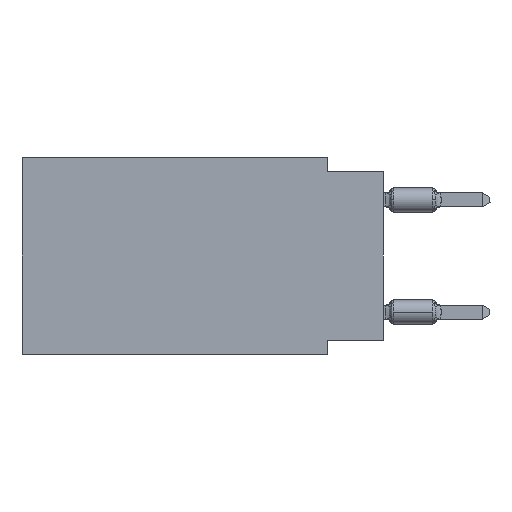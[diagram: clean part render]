
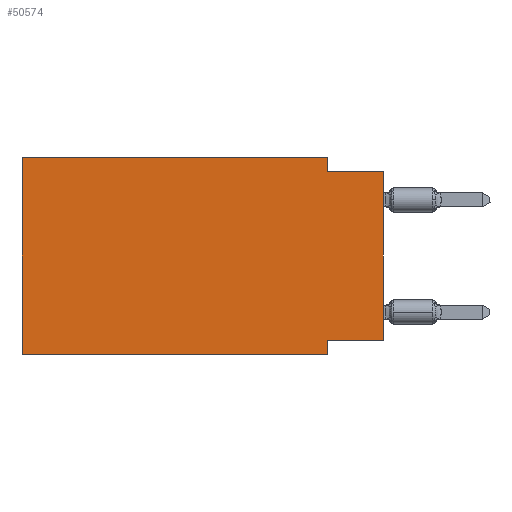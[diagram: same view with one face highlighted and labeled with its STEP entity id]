
A CAD part, left-side view. The second image highlights one B-rep face of the part: STEP entity #50574.
In plain terms, the highlighted planar face has unit normal (-1, 0, 0).
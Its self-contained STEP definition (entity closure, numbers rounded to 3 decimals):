
#2244 = VECTOR ( 'NONE', #19840, 1000. ) ;
#3026 = AXIS2_PLACEMENT_3D ( 'NONE', #25866, #55266, #50048 ) ;
#5818 = VERTEX_POINT ( 'NONE', #38947 ) ;
#6090 = DIRECTION ( 'NONE',  ( 0., 0., -1. ) ) ;
#6147 = ORIENTED_EDGE ( 'NONE', *, *, #39182, .F. ) ;
#7715 = EDGE_CURVE ( 'NONE', #68436, #34919, #61550, .T. ) ;
#7778 = VERTEX_POINT ( 'NONE', #38865 ) ;
#8231 = EDGE_CURVE ( 'NONE', #7778, #45000, #68686, .T. ) ;
#8926 = LINE ( 'NONE', #21599, #73499 ) ;
#9956 = CARTESIAN_POINT ( 'NONE',  ( 0., 0., -8.255 ) ) ;
#10507 = DIRECTION ( 'NONE',  ( 0., 1., 0. ) ) ;
#10569 = LINE ( 'NONE', #57133, #27972 ) ;
#10819 = LINE ( 'NONE', #20940, #14606 ) ;
#11310 = EDGE_CURVE ( 'NONE', #34919, #45000, #65997, .T. ) ;
#12389 = CARTESIAN_POINT ( 'NONE',  ( 0., 0., -0.635 ) ) ;
#12663 = VECTOR ( 'NONE', #46762, 1000. ) ;
#14606 = VECTOR ( 'NONE', #15705, 1000. ) ;
#14997 = CARTESIAN_POINT ( 'NONE',  ( 0., 2.54, -8.89 ) ) ;
#15705 = DIRECTION ( 'NONE',  ( 0., 0., 1. ) ) ;
#18002 = EDGE_CURVE ( 'NONE', #7778, #5818, #10819, .T. ) ;
#18494 = EDGE_LOOP ( 'NONE', ( #29367, #34802, #73128, #6147, #46559, #66873, #67844, #57927 ) ) ;
#19840 = DIRECTION ( 'NONE',  ( 0., 0., -1. ) ) ;
#20940 = CARTESIAN_POINT ( 'NONE',  ( 0., 16.383, 0. ) ) ;
#21599 = CARTESIAN_POINT ( 'NONE',  ( 0., 0., 0. ) ) ;
#25866 = CARTESIAN_POINT ( 'NONE',  ( 0., 16.383, 0. ) ) ;
#27972 = VECTOR ( 'NONE', #6090, 1000. ) ;
#28080 = VECTOR ( 'NONE', #10507, 1000. ) ;
#28138 = VECTOR ( 'NONE', #39298, 1000. ) ;
#29367 = ORIENTED_EDGE ( 'NONE', *, *, #40672, .T. ) ;
#34475 = CARTESIAN_POINT ( 'NONE',  ( 0., 16.383, -8.89 ) ) ;
#34802 = ORIENTED_EDGE ( 'NONE', *, *, #45040, .F. ) ;
#34919 = VERTEX_POINT ( 'NONE', #46418 ) ;
#35697 = VERTEX_POINT ( 'NONE', #38831 ) ;
#37161 = DIRECTION ( 'NONE',  ( 0., -1., 0. ) ) ;
#38137 = CARTESIAN_POINT ( 'NONE',  ( 0., 0., -8.255 ) ) ;
#38831 = CARTESIAN_POINT ( 'NONE',  ( 0., 2.54, 0. ) ) ;
#38865 = CARTESIAN_POINT ( 'NONE',  ( 0., 16.383, -8.89 ) ) ;
#38895 = FACE_OUTER_BOUND ( 'NONE', #18494, .T. ) ;
#38947 = CARTESIAN_POINT ( 'NONE',  ( 0., 16.383, 0. ) ) ;
#39182 = EDGE_CURVE ( 'NONE', #5818, #35697, #64351, .T. ) ;
#39298 = DIRECTION ( 'NONE',  ( 0., -1., 0. ) ) ;
#40672 = EDGE_CURVE ( 'NONE', #68436, #45465, #8926, .T. ) ;
#45000 = VERTEX_POINT ( 'NONE', #52355 ) ;
#45040 = EDGE_CURVE ( 'NONE', #68903, #45465, #46406, .T. ) ;
#45465 = VERTEX_POINT ( 'NONE', #12389 ) ;
#45671 = CARTESIAN_POINT ( 'NONE',  ( 0., 0., -0.635 ) ) ;
#46406 = LINE ( 'NONE', #45671, #12663 ) ;
#46418 = CARTESIAN_POINT ( 'NONE',  ( 0., 2.54, -8.255 ) ) ;
#46559 = ORIENTED_EDGE ( 'NONE', *, *, #18002, .F. ) ;
#46762 = DIRECTION ( 'NONE',  ( 0., -1., 0. ) ) ;
#48316 = CARTESIAN_POINT ( 'NONE',  ( 0., 16.383, 0. ) ) ;
#50048 = DIRECTION ( 'NONE',  ( 0., 0., -1. ) ) ;
#50574 = ADVANCED_FACE ( 'NONE', ( #38895 ), #66065, .F. ) ;
#52355 = CARTESIAN_POINT ( 'NONE',  ( 0., 2.54, -8.89 ) ) ;
#54761 = DIRECTION ( 'NONE',  ( 0., 0., 1. ) ) ;
#55266 = DIRECTION ( 'NONE',  ( 1., 0., 0. ) ) ;
#56053 = CARTESIAN_POINT ( 'NONE',  ( 0., 2.54, -0.635 ) ) ;
#57133 = CARTESIAN_POINT ( 'NONE',  ( 0., 2.54, 0. ) ) ;
#57927 = ORIENTED_EDGE ( 'NONE', *, *, #7715, .F. ) ;
#60424 = VECTOR ( 'NONE', #37161, 1000. ) ;
#61550 = LINE ( 'NONE', #38137, #28080 ) ;
#64351 = LINE ( 'NONE', #48316, #60424 ) ;
#65997 = LINE ( 'NONE', #14997, #2244 ) ;
#66065 = PLANE ( 'NONE',  #3026 ) ;
#66873 = ORIENTED_EDGE ( 'NONE', *, *, #8231, .T. ) ;
#67844 = ORIENTED_EDGE ( 'NONE', *, *, #11310, .F. ) ;
#68436 = VERTEX_POINT ( 'NONE', #9956 ) ;
#68686 = LINE ( 'NONE', #34475, #28138 ) ;
#68903 = VERTEX_POINT ( 'NONE', #56053 ) ;
#72987 = EDGE_CURVE ( 'NONE', #35697, #68903, #10569, .T. ) ;
#73128 = ORIENTED_EDGE ( 'NONE', *, *, #72987, .F. ) ;
#73499 = VECTOR ( 'NONE', #54761, 1000. ) ;
